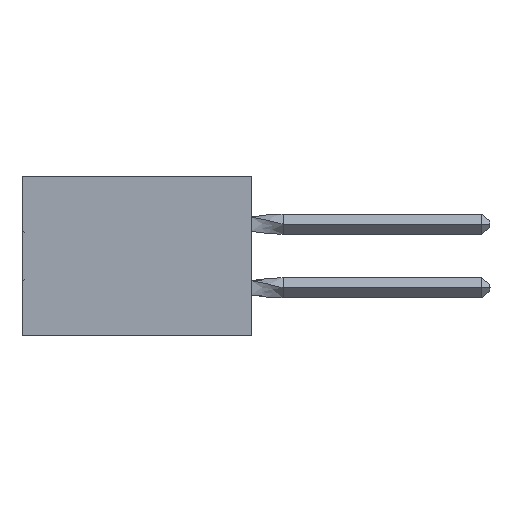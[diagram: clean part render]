
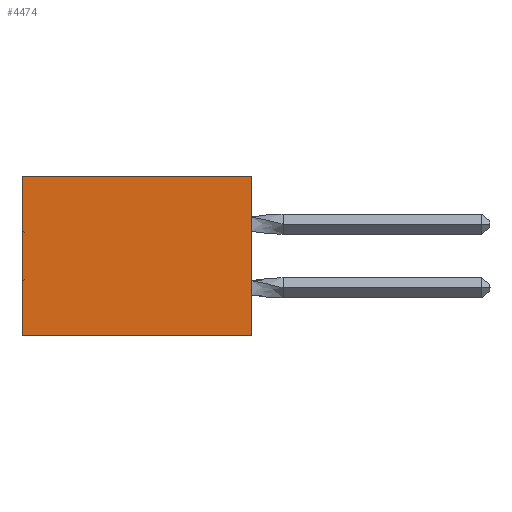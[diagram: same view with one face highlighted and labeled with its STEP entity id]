
A CAD part, left-side view. The second image highlights one B-rep face of the part: STEP entity #4474.
In plain terms, the highlighted planar face has unit normal (-1, 0, 0).
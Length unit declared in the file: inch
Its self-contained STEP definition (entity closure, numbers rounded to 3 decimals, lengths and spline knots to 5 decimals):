
#201 = AXIS2_PLACEMENT_3D ( 'NONE', #40959, #14476, #1274 ) ;
#319 = CARTESIAN_POINT ( 'NONE',  ( 0.305, 0., 0. ) ) ;
#764 = DIRECTION ( 'NONE',  ( 0., 0., -1. ) ) ;
#1274 = DIRECTION ( 'NONE',  ( 0., 0., -1. ) ) ;
#1710 = VERTEX_POINT ( 'NONE', #19632 ) ;
#2957 = EDGE_CURVE ( 'NONE', #48690, #21941, #28235, .T. ) ;
#4474 = ADVANCED_FACE ( 'NONE', ( #19014 ), #9853, .F. ) ;
#4715 = EDGE_CURVE ( 'NONE', #1710, #21941, #42699, .T. ) ;
#5535 = VERTEX_POINT ( 'NONE', #319 ) ;
#8080 = CARTESIAN_POINT ( 'NONE',  ( 0.305, 0.72, -0.5 ) ) ;
#9853 = PLANE ( 'NONE',  #201 ) ;
#11285 = VECTOR ( 'NONE', #52955, 39.37008 ) ;
#13002 = LINE ( 'NONE', #49993, #38780 ) ;
#14476 = DIRECTION ( 'NONE',  ( 1., 0., 0. ) ) ;
#19014 = FACE_OUTER_BOUND ( 'NONE', #42381, .T. ) ;
#19632 = CARTESIAN_POINT ( 'NONE',  ( 0.305, 0.72, 0. ) ) ;
#21362 = CARTESIAN_POINT ( 'NONE',  ( 0.305, 0., 0. ) ) ;
#21441 = EDGE_CURVE ( 'NONE', #5535, #1710, #28598, .T. ) ;
#21941 = VERTEX_POINT ( 'NONE', #30318 ) ;
#22627 = VECTOR ( 'NONE', #35810, 39.37008 ) ;
#23335 = ORIENTED_EDGE ( 'NONE', *, *, #51729, .F. ) ;
#28235 = LINE ( 'NONE', #36385, #22627 ) ;
#28448 = ORIENTED_EDGE ( 'NONE', *, *, #2957, .F. ) ;
#28598 = LINE ( 'NONE', #21362, #11285 ) ;
#30318 = CARTESIAN_POINT ( 'NONE',  ( 0.305, 0.72, -0.5 ) ) ;
#35810 = DIRECTION ( 'NONE',  ( 0., 1., 0. ) ) ;
#36124 = ORIENTED_EDGE ( 'NONE', *, *, #4715, .T. ) ;
#36235 = CARTESIAN_POINT ( 'NONE',  ( 0.305, 0., -0.5 ) ) ;
#36385 = CARTESIAN_POINT ( 'NONE',  ( 0.305, 0., -0.5 ) ) ;
#38780 = VECTOR ( 'NONE', #764, 39.37008 ) ;
#40959 = CARTESIAN_POINT ( 'NONE',  ( 0.305, 0., -0.5 ) ) ;
#42381 = EDGE_LOOP ( 'NONE', ( #36124, #28448, #23335, #51605 ) ) ;
#42699 = LINE ( 'NONE', #8080, #57360 ) ;
#43641 = DIRECTION ( 'NONE',  ( 0., 0., -1. ) ) ;
#48690 = VERTEX_POINT ( 'NONE', #36235 ) ;
#49993 = CARTESIAN_POINT ( 'NONE',  ( 0.305, 0., -0.5 ) ) ;
#51605 = ORIENTED_EDGE ( 'NONE', *, *, #21441, .T. ) ;
#51729 = EDGE_CURVE ( 'NONE', #5535, #48690, #13002, .T. ) ;
#52955 = DIRECTION ( 'NONE',  ( 0., 1., 0. ) ) ;
#57360 = VECTOR ( 'NONE', #43641, 39.37008 ) ;
